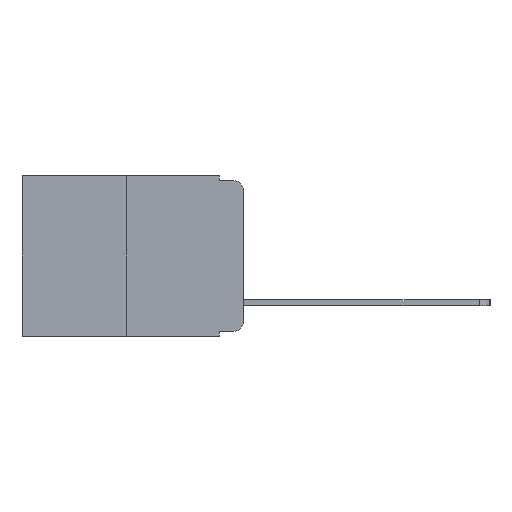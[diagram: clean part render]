
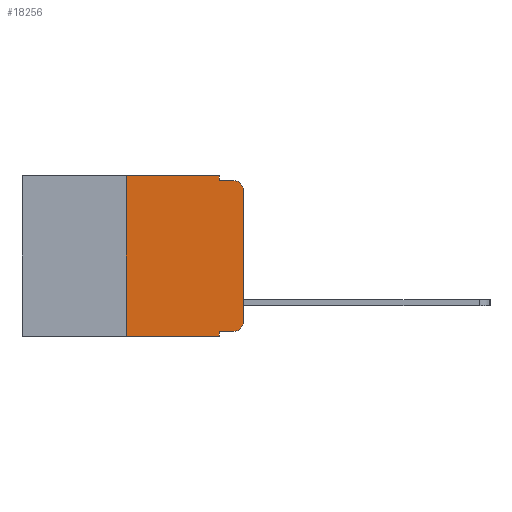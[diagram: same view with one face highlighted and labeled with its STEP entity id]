
A CAD part, left-side view. The second image highlights one B-rep face of the part: STEP entity #18256.
In plain terms, the highlighted planar face has unit normal (-1, 0, 0).
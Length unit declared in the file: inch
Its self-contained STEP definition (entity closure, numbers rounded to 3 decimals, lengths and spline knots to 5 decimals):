
#544 = EDGE_CURVE ( 'NONE', #1225, #19327, #7156, .T. ) ;
#575 = EDGE_CURVE ( 'NONE', #19327, #5828, #10695, .T. ) ;
#579 = EDGE_CURVE ( 'NONE', #4769, #5828, #6169, .T. ) ;
#594 = VECTOR ( 'NONE', #4952, 39.37008 ) ;
#603 = EDGE_CURVE ( 'NONE', #11673, #4769, #9329, .T. ) ;
#606 = EDGE_CURVE ( 'NONE', #19301, #7449, #1651, .T. ) ;
#641 = EDGE_CURVE ( 'NONE', #7386, #18536, #1158, .T. ) ;
#643 = EDGE_CURVE ( 'NONE', #7386, #4805, #12300, .T. ) ;
#646 = EDGE_CURVE ( 'NONE', #4805, #1225, #4747, .T. ) ;
#984 = ORIENTED_EDGE ( 'NONE', *, *, #1838, .T. ) ;
#1158 = LINE ( 'NONE', #3396, #594 ) ;
#1197 = CARTESIAN_POINT ( 'NONE',  ( 0., 0.473, -0.343 ) ) ;
#1225 = VERTEX_POINT ( 'NONE', #6419 ) ;
#1651 = LINE ( 'NONE', #12252, #9795 ) ;
#1752 = CARTESIAN_POINT ( 'NONE',  ( 0., 0.02, -0.01 ) ) ;
#1814 = DIRECTION ( 'NONE',  ( 0., 0., 1. ) ) ;
#1838 = EDGE_CURVE ( 'NONE', #19301, #18536, #2560, .T. ) ;
#1995 = EDGE_CURVE ( 'NONE', #7449, #11673, #11795, .T. ) ;
#2560 = LINE ( 'NONE', #1197, #6638 ) ;
#3396 = CARTESIAN_POINT ( 'NONE',  ( 0., 0.051, 0. ) ) ;
#4274 = VECTOR ( 'NONE', #16751, 39.37008 ) ;
#4736 = DIRECTION ( 'NONE',  ( -1., 0., 0. ) ) ;
#4747 = CIRCLE ( 'NONE', #11549, 0.02 ) ;
#4769 = VERTEX_POINT ( 'NONE', #4966 ) ;
#4805 = VERTEX_POINT ( 'NONE', #19304 ) ;
#4952 = DIRECTION ( 'NONE',  ( 0., 0., -1. ) ) ;
#4966 = CARTESIAN_POINT ( 'NONE',  ( 0., 0.051, -0.01 ) ) ;
#5025 = CARTESIAN_POINT ( 'NONE',  ( 0., 0.02, -0.313 ) ) ;
#5241 = VECTOR ( 'NONE', #9461, 39.37008 ) ;
#5353 = ORIENTED_EDGE ( 'NONE', *, *, #603, .F. ) ;
#5828 = VERTEX_POINT ( 'NONE', #1752 ) ;
#5912 = CARTESIAN_POINT ( 'NONE',  ( 0., 0., -0.03 ) ) ;
#6169 = LINE ( 'NONE', #19314, #17420 ) ;
#6419 = CARTESIAN_POINT ( 'NONE',  ( 0., 0., -0.313 ) ) ;
#6498 = AXIS2_PLACEMENT_3D ( 'NONE', #13730, #4736, #15162 ) ;
#6547 = CARTESIAN_POINT ( 'NONE',  ( 0., 0.051, -0.333 ) ) ;
#6554 = DIRECTION ( 'NONE',  ( 0., 0., -1. ) ) ;
#6638 = VECTOR ( 'NONE', #6769, 39.37008 ) ;
#6677 = VECTOR ( 'NONE', #7698, 39.37008 ) ;
#6769 = DIRECTION ( 'NONE',  ( 0., -1., 0. ) ) ;
#6988 = ORIENTED_EDGE ( 'NONE', *, *, #544, .T. ) ;
#7156 = LINE ( 'NONE', #12121, #6677 ) ;
#7386 = VERTEX_POINT ( 'NONE', #6547 ) ;
#7449 = VERTEX_POINT ( 'NONE', #16876 ) ;
#7463 = ORIENTED_EDGE ( 'NONE', *, *, #579, .F. ) ;
#7698 = DIRECTION ( 'NONE',  ( 0., 0., 1. ) ) ;
#8699 = ORIENTED_EDGE ( 'NONE', *, *, #641, .F. ) ;
#8929 = DIRECTION ( 'NONE',  ( 0., 0., -1. ) ) ;
#8957 = ORIENTED_EDGE ( 'NONE', *, *, #575, .T. ) ;
#9329 = LINE ( 'NONE', #9985, #5241 ) ;
#9461 = DIRECTION ( 'NONE',  ( 0., 0., -1. ) ) ;
#9795 = VECTOR ( 'NONE', #1814, 39.37008 ) ;
#9908 = ORIENTED_EDGE ( 'NONE', *, *, #606, .F. ) ;
#9985 = CARTESIAN_POINT ( 'NONE',  ( 0., 0.051, 0. ) ) ;
#10695 = CIRCLE ( 'NONE', #6498, 0.02 ) ;
#10837 = DIRECTION ( 'NONE',  ( 0., -1., 0. ) ) ;
#11549 = AXIS2_PLACEMENT_3D ( 'NONE', #5025, #15419, #6554 ) ;
#11673 = VERTEX_POINT ( 'NONE', #17589 ) ;
#11795 = LINE ( 'NONE', #12823, #15639 ) ;
#12121 = CARTESIAN_POINT ( 'NONE',  ( 0., 0., 0. ) ) ;
#12252 = CARTESIAN_POINT ( 'NONE',  ( 0., 0.25, 0. ) ) ;
#12300 = LINE ( 'NONE', #15365, #4274 ) ;
#12407 = FACE_OUTER_BOUND ( 'NONE', #14620, .T. ) ;
#12464 = CARTESIAN_POINT ( 'NONE',  ( 0., 0.051, -0.343 ) ) ;
#12823 = CARTESIAN_POINT ( 'NONE',  ( 0., 0.473, 0. ) ) ;
#13301 = CARTESIAN_POINT ( 'NONE',  ( 0., 0.473, 0. ) ) ;
#13334 = CARTESIAN_POINT ( 'NONE',  ( 0., 0.25, -0.343 ) ) ;
#13661 = DIRECTION ( 'NONE',  ( 0., -1., 0. ) ) ;
#13730 = CARTESIAN_POINT ( 'NONE',  ( 0., 0.02, -0.03 ) ) ;
#14620 = EDGE_LOOP ( 'NONE', ( #6988, #8957, #7463, #5353, #17090, #9908, #984, #8699, #18820, #18389 ) ) ;
#15162 = DIRECTION ( 'NONE',  ( 0., 0., -1. ) ) ;
#15365 = CARTESIAN_POINT ( 'NONE',  ( 0., 0.051, -0.333 ) ) ;
#15419 = DIRECTION ( 'NONE',  ( -1., 0., 0. ) ) ;
#15639 = VECTOR ( 'NONE', #10837, 39.37008 ) ;
#16143 = PLANE ( 'NONE',  #17737 ) ;
#16751 = DIRECTION ( 'NONE',  ( 0., -1., 0. ) ) ;
#16876 = CARTESIAN_POINT ( 'NONE',  ( 0., 0.25, 0. ) ) ;
#17090 = ORIENTED_EDGE ( 'NONE', *, *, #1995, .F. ) ;
#17420 = VECTOR ( 'NONE', #13661, 39.37008 ) ;
#17566 = DIRECTION ( 'NONE',  ( 1., 0., 0. ) ) ;
#17589 = CARTESIAN_POINT ( 'NONE',  ( 0., 0.051, 0. ) ) ;
#17737 = AXIS2_PLACEMENT_3D ( 'NONE', #13301, #17566, #8929 ) ;
#18256 = ADVANCED_FACE ( 'NONE', ( #12407 ), #16143, .F. ) ;
#18389 = ORIENTED_EDGE ( 'NONE', *, *, #646, .T. ) ;
#18536 = VERTEX_POINT ( 'NONE', #12464 ) ;
#18820 = ORIENTED_EDGE ( 'NONE', *, *, #643, .T. ) ;
#19301 = VERTEX_POINT ( 'NONE', #13334 ) ;
#19304 = CARTESIAN_POINT ( 'NONE',  ( 0., 0.02, -0.333 ) ) ;
#19314 = CARTESIAN_POINT ( 'NONE',  ( 0., 0.051, -0.01 ) ) ;
#19327 = VERTEX_POINT ( 'NONE', #5912 ) ;
